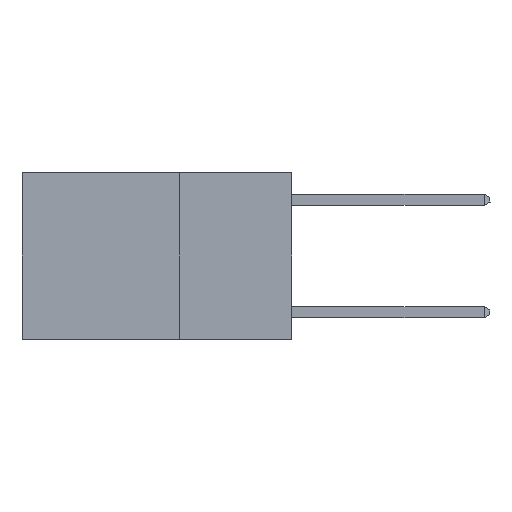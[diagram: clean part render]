
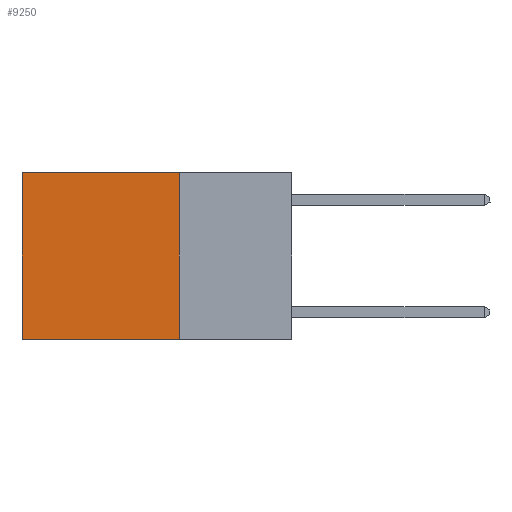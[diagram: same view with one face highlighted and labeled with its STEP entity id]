
A CAD part, left-side view. The second image highlights one B-rep face of the part: STEP entity #9250.
In plain terms, the highlighted planar face has unit normal (-1, 0, 0).
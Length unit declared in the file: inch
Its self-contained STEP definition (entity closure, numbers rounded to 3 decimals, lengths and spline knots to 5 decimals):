
#1178 = LINE ( 'NONE', #30218, #25192 ) ;
#1865 = DIRECTION ( 'NONE',  ( 0., 1., 0. ) ) ;
#2667 = CARTESIAN_POINT ( 'NONE',  ( 0.2625, 0.6, -0.37 ) ) ;
#3090 = VECTOR ( 'NONE', #6322, 39.37008 ) ;
#3505 = VECTOR ( 'NONE', #30644, 39.37008 ) ;
#3774 = ORIENTED_EDGE ( 'NONE', *, *, #20419, .F. ) ;
#5186 = CARTESIAN_POINT ( 'NONE',  ( 0.2625, 0.25, -0.37 ) ) ;
#6292 = EDGE_CURVE ( 'NONE', #9079, #14340, #26023, .T. ) ;
#6322 = DIRECTION ( 'NONE',  ( 0., 0., -1. ) ) ;
#9079 = VERTEX_POINT ( 'NONE', #27663 ) ;
#9126 = ORIENTED_EDGE ( 'NONE', *, *, #10052, .T. ) ;
#9182 = EDGE_CURVE ( 'NONE', #9377, #15501, #1178, .T. ) ;
#9250 = ADVANCED_FACE ( 'NONE', ( #16881 ), #9578, .F. ) ;
#9288 = ORIENTED_EDGE ( 'NONE', *, *, #6292, .T. ) ;
#9377 = VERTEX_POINT ( 'NONE', #5186 ) ;
#9578 = PLANE ( 'NONE',  #10099 ) ;
#9874 = CARTESIAN_POINT ( 'NONE',  ( 0.2625, 0.6, 0. ) ) ;
#10052 = EDGE_CURVE ( 'NONE', #14340, #15501, #16479, .T. ) ;
#10099 = AXIS2_PLACEMENT_3D ( 'NONE', #12039, #28241, #14476 ) ;
#11762 = EDGE_LOOP ( 'NONE', ( #9126, #19307, #3774, #9288 ) ) ;
#12039 = CARTESIAN_POINT ( 'NONE',  ( 0.2625, 0.25, 0. ) ) ;
#14340 = VERTEX_POINT ( 'NONE', #24700 ) ;
#14476 = DIRECTION ( 'NONE',  ( 0., 0., -1. ) ) ;
#15501 = VERTEX_POINT ( 'NONE', #2667 ) ;
#16479 = LINE ( 'NONE', #9874, #3505 ) ;
#16820 = LINE ( 'NONE', #25248, #3090 ) ;
#16881 = FACE_OUTER_BOUND ( 'NONE', #11762, .T. ) ;
#19307 = ORIENTED_EDGE ( 'NONE', *, *, #9182, .F. ) ;
#20419 = EDGE_CURVE ( 'NONE', #9079, #9377, #16820, .T. ) ;
#20450 = CARTESIAN_POINT ( 'NONE',  ( 0.2625, 0.25, 0. ) ) ;
#21453 = VECTOR ( 'NONE', #27253, 39.37008 ) ;
#24700 = CARTESIAN_POINT ( 'NONE',  ( 0.2625, 0.6, 0. ) ) ;
#25192 = VECTOR ( 'NONE', #1865, 39.37008 ) ;
#25248 = CARTESIAN_POINT ( 'NONE',  ( 0.2625, 0.25, 0. ) ) ;
#26023 = LINE ( 'NONE', #20450, #21453 ) ;
#27253 = DIRECTION ( 'NONE',  ( 0., 1., 0. ) ) ;
#27663 = CARTESIAN_POINT ( 'NONE',  ( 0.2625, 0.25, 0. ) ) ;
#28241 = DIRECTION ( 'NONE',  ( 1., 0., 0. ) ) ;
#30218 = CARTESIAN_POINT ( 'NONE',  ( 0.2625, 0.25, -0.37 ) ) ;
#30644 = DIRECTION ( 'NONE',  ( 0., 0., -1. ) ) ;
